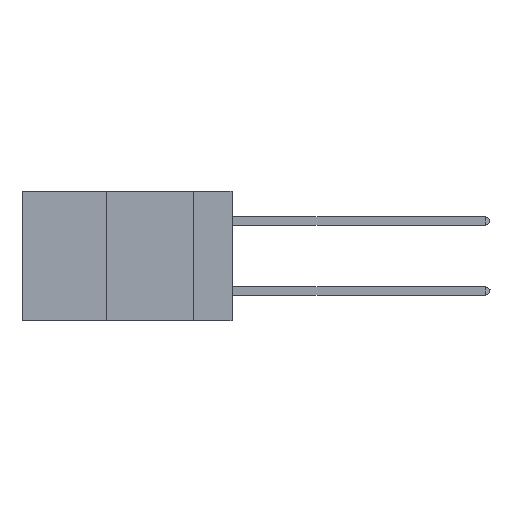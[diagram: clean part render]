
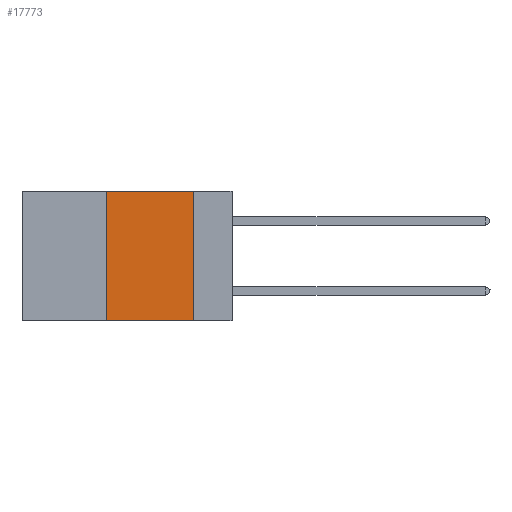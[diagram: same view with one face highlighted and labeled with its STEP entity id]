
A CAD part, left-side view. The second image highlights one B-rep face of the part: STEP entity #17773.
In plain terms, the highlighted planar face has unit normal (-1, 0, 0).
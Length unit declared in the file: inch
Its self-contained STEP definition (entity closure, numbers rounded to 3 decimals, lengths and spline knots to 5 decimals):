
#642 = ORIENTED_EDGE ( 'NONE', *, *, #6876, .F. ) ;
#2705 = DIRECTION ( 'NONE',  ( 0., 0., 1. ) ) ;
#6585 = DIRECTION ( 'NONE',  ( 0., 0., -1. ) ) ;
#6876 = EDGE_CURVE ( 'NONE', #10472, #34503, #30727, .T. ) ;
#7180 = DIRECTION ( 'NONE',  ( 1., 0., 0. ) ) ;
#7878 = VECTOR ( 'NONE', #6585, 39.37008 ) ;
#10091 = LINE ( 'NONE', #29057, #27157 ) ;
#10472 = VERTEX_POINT ( 'NONE', #34474 ) ;
#10524 = ORIENTED_EDGE ( 'NONE', *, *, #31110, .F. ) ;
#10539 = EDGE_CURVE ( 'NONE', #30257, #16108, #21094, .T. ) ;
#10540 = VECTOR ( 'NONE', #24342, 39.37008 ) ;
#10702 = CARTESIAN_POINT ( 'NONE',  ( 0., 0.11, -0.37 ) ) ;
#12041 = FACE_OUTER_BOUND ( 'NONE', #21318, .T. ) ;
#15156 = CARTESIAN_POINT ( 'NONE',  ( 0., 0.11, 0. ) ) ;
#16015 = CARTESIAN_POINT ( 'NONE',  ( 0., 0.6, 0. ) ) ;
#16108 = VERTEX_POINT ( 'NONE', #10702 ) ;
#17403 = CARTESIAN_POINT ( 'NONE',  ( 0., 0.6, -0.37 ) ) ;
#17718 = ORIENTED_EDGE ( 'NONE', *, *, #36597, .F. ) ;
#17773 = ADVANCED_FACE ( 'NONE', ( #12041 ), #33464, .F. ) ;
#19147 = AXIS2_PLACEMENT_3D ( 'NONE', #16015, #7180, #36796 ) ;
#20543 = CARTESIAN_POINT ( 'NONE',  ( 0., 0.11, 0. ) ) ;
#21094 = LINE ( 'NONE', #17403, #10540 ) ;
#21318 = EDGE_LOOP ( 'NONE', ( #10524, #642, #17718, #34066 ) ) ;
#22766 = DIRECTION ( 'NONE',  ( 0., -1., 0. ) ) ;
#24342 = DIRECTION ( 'NONE',  ( 0., -1., 0. ) ) ;
#27157 = VECTOR ( 'NONE', #2705, 39.37008 ) ;
#29057 = CARTESIAN_POINT ( 'NONE',  ( 0., 0.36, 0. ) ) ;
#30257 = VERTEX_POINT ( 'NONE', #34807 ) ;
#30727 = LINE ( 'NONE', #30917, #33482 ) ;
#30917 = CARTESIAN_POINT ( 'NONE',  ( 0., 0.6, 0. ) ) ;
#31110 = EDGE_CURVE ( 'NONE', #34503, #16108, #35473, .T. ) ;
#33464 = PLANE ( 'NONE',  #19147 ) ;
#33482 = VECTOR ( 'NONE', #22766, 39.37008 ) ;
#34066 = ORIENTED_EDGE ( 'NONE', *, *, #10539, .T. ) ;
#34474 = CARTESIAN_POINT ( 'NONE',  ( 0., 0.36, 0. ) ) ;
#34503 = VERTEX_POINT ( 'NONE', #20543 ) ;
#34807 = CARTESIAN_POINT ( 'NONE',  ( 0., 0.36, -0.37 ) ) ;
#35473 = LINE ( 'NONE', #15156, #7878 ) ;
#36597 = EDGE_CURVE ( 'NONE', #30257, #10472, #10091, .T. ) ;
#36796 = DIRECTION ( 'NONE',  ( 0., 0., -1. ) ) ;
